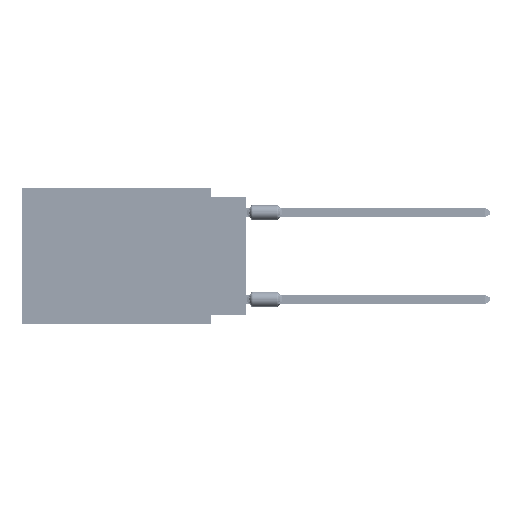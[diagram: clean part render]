
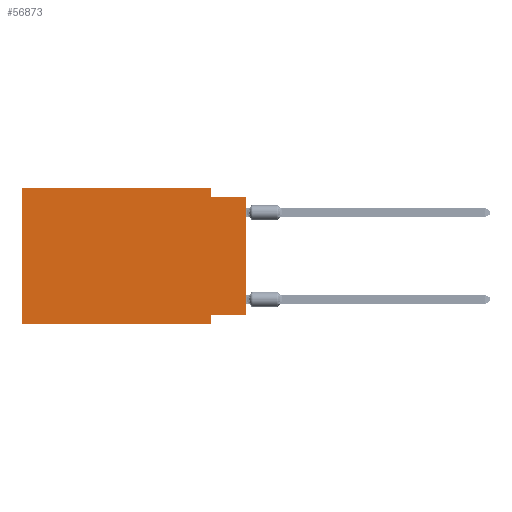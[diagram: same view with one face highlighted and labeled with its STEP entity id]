
A CAD part, left-side view. The second image highlights one B-rep face of the part: STEP entity #56873.
In plain terms, the highlighted planar face has unit normal (-1, 0, 0).
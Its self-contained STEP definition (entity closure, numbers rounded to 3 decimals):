
#42 = ORIENTED_EDGE ( 'NONE', *, *, #1195, .F. ) ;
#482 = CARTESIAN_POINT ( 'NONE',  ( 0., 16.383, 0. ) ) ;
#1195 = EDGE_CURVE ( 'NONE', #27920, #3673, #49242, .T. ) ;
#2190 = CARTESIAN_POINT ( 'NONE',  ( 0., 16.383, -9.906 ) ) ;
#2845 = CARTESIAN_POINT ( 'NONE',  ( 0., 16.383, 0. ) ) ;
#3673 = VERTEX_POINT ( 'NONE', #16012 ) ;
#6525 = EDGE_CURVE ( 'NONE', #72327, #27920, #14041, .T. ) ;
#6812 = VECTOR ( 'NONE', #52738, 1000. ) ;
#7324 = CARTESIAN_POINT ( 'NONE',  ( 0., 2.54, 0. ) ) ;
#8246 = DIRECTION ( 'NONE',  ( 0., 0., -1. ) ) ;
#8448 = EDGE_CURVE ( 'NONE', #62177, #35343, #47717, .T. ) ;
#9391 = DIRECTION ( 'NONE',  ( 0., 0., -1. ) ) ;
#14041 = LINE ( 'NONE', #37471, #50825 ) ;
#14396 = CARTESIAN_POINT ( 'NONE',  ( 0., 2.54, -9.906 ) ) ;
#16012 = CARTESIAN_POINT ( 'NONE',  ( 0., 0., -0.635 ) ) ;
#16174 = ORIENTED_EDGE ( 'NONE', *, *, #73843, .T. ) ;
#18288 = LINE ( 'NONE', #50724, #72855 ) ;
#19486 = VECTOR ( 'NONE', #71558, 1000. ) ;
#19571 = EDGE_CURVE ( 'NONE', #25631, #62177, #75910, .T. ) ;
#22123 = VERTEX_POINT ( 'NONE', #482 ) ;
#24048 = DIRECTION ( 'NONE',  ( 0., 0., 1. ) ) ;
#24922 = DIRECTION ( 'NONE',  ( 1., 0., 0. ) ) ;
#25631 = VERTEX_POINT ( 'NONE', #65023 ) ;
#25938 = LINE ( 'NONE', #2845, #61110 ) ;
#27757 = EDGE_CURVE ( 'NONE', #71719, #35343, #33478, .T. ) ;
#27920 = VERTEX_POINT ( 'NONE', #41154 ) ;
#30089 = VECTOR ( 'NONE', #47070, 1000. ) ;
#30692 = PLANE ( 'NONE',  #33357 ) ;
#33357 = AXIS2_PLACEMENT_3D ( 'NONE', #50546, #24922, #9391 ) ;
#33478 = LINE ( 'NONE', #63845, #67050 ) ;
#35343 = VERTEX_POINT ( 'NONE', #14396 ) ;
#37427 = ORIENTED_EDGE ( 'NONE', *, *, #27757, .T. ) ;
#37471 = CARTESIAN_POINT ( 'NONE',  ( 0., 2.54, 0. ) ) ;
#40986 = DIRECTION ( 'NONE',  ( 0., 0., 1. ) ) ;
#41154 = CARTESIAN_POINT ( 'NONE',  ( 0., 2.54, -0.635 ) ) ;
#43676 = EDGE_LOOP ( 'NONE', ( #16174, #42, #72304, #71735, #47021, #37427, #56967, #61374 ) ) ;
#44109 = CARTESIAN_POINT ( 'NONE',  ( 0., 2.54, -9.271 ) ) ;
#45107 = EDGE_CURVE ( 'NONE', #22123, #72327, #25938, .T. ) ;
#45790 = DIRECTION ( 'NONE',  ( 0., -1., 0. ) ) ;
#47021 = ORIENTED_EDGE ( 'NONE', *, *, #70137, .F. ) ;
#47070 = DIRECTION ( 'NONE',  ( 0., 1., 0. ) ) ;
#47717 = LINE ( 'NONE', #65020, #6812 ) ;
#47879 = LINE ( 'NONE', #65561, #69564 ) ;
#49242 = LINE ( 'NONE', #66543, #19486 ) ;
#50546 = CARTESIAN_POINT ( 'NONE',  ( 0., 16.383, 0. ) ) ;
#50724 = CARTESIAN_POINT ( 'NONE',  ( 0., 16.383, 0. ) ) ;
#50825 = VECTOR ( 'NONE', #8246, 1000. ) ;
#52738 = DIRECTION ( 'NONE',  ( 0., 0., -1. ) ) ;
#56873 = ADVANCED_FACE ( 'NONE', ( #60661 ), #30692, .F. ) ;
#56967 = ORIENTED_EDGE ( 'NONE', *, *, #8448, .F. ) ;
#60549 = DIRECTION ( 'NONE',  ( 0., -1., 0. ) ) ;
#60661 = FACE_OUTER_BOUND ( 'NONE', #43676, .T. ) ;
#61110 = VECTOR ( 'NONE', #60549, 1000. ) ;
#61374 = ORIENTED_EDGE ( 'NONE', *, *, #19571, .F. ) ;
#62177 = VERTEX_POINT ( 'NONE', #44109 ) ;
#63845 = CARTESIAN_POINT ( 'NONE',  ( 0., 16.383, -9.906 ) ) ;
#64738 = CARTESIAN_POINT ( 'NONE',  ( 0., 0., -9.271 ) ) ;
#65020 = CARTESIAN_POINT ( 'NONE',  ( 0., 2.54, -9.906 ) ) ;
#65023 = CARTESIAN_POINT ( 'NONE',  ( 0., 0., -9.271 ) ) ;
#65561 = CARTESIAN_POINT ( 'NONE',  ( 0., 0., 0. ) ) ;
#66543 = CARTESIAN_POINT ( 'NONE',  ( 0., 0., -0.635 ) ) ;
#67050 = VECTOR ( 'NONE', #45790, 1000. ) ;
#69564 = VECTOR ( 'NONE', #24048, 1000. ) ;
#70137 = EDGE_CURVE ( 'NONE', #71719, #22123, #18288, .T. ) ;
#71558 = DIRECTION ( 'NONE',  ( 0., -1., 0. ) ) ;
#71719 = VERTEX_POINT ( 'NONE', #2190 ) ;
#71735 = ORIENTED_EDGE ( 'NONE', *, *, #45107, .F. ) ;
#72304 = ORIENTED_EDGE ( 'NONE', *, *, #6525, .F. ) ;
#72327 = VERTEX_POINT ( 'NONE', #7324 ) ;
#72855 = VECTOR ( 'NONE', #40986, 1000. ) ;
#73843 = EDGE_CURVE ( 'NONE', #25631, #3673, #47879, .T. ) ;
#75910 = LINE ( 'NONE', #64738, #30089 ) ;
